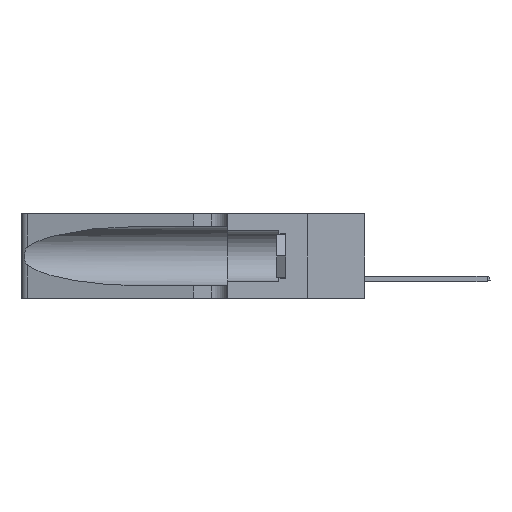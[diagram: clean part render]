
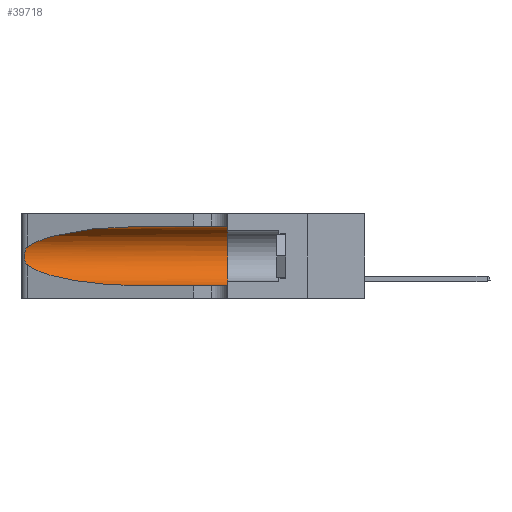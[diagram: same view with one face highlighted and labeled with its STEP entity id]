
A CAD part, left-side view. The second image highlights one B-rep face of the part: STEP entity #39718.
In plain terms, the highlighted cylindrical face has radius 3.308 mm (diameter 6.617 mm), a partial arc.
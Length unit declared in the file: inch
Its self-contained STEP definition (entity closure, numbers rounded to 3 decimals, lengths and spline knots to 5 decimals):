
#500 = VECTOR ( 'NONE', #27007, 39.37008 ) ;
#865 = EDGE_CURVE ( 'NONE', #6688, #7810, #17325, .T. ) ;
#954 = ORIENTED_EDGE ( 'NONE', *, *, #17991, .F. ) ;
#1608 = CARTESIAN_POINT ( 'NONE',  ( 0.1305, 0.72297, 0.05475 ) ) ;
#1954 = ORIENTED_EDGE ( 'NONE', *, *, #3819, .F. ) ;
#2489 = CARTESIAN_POINT ( 'NONE',  ( 0.26018, 1.23835, 0.19895 ) ) ;
#2500 = CARTESIAN_POINT ( 'NONE',  ( 0.1305, 0.72297, 0.31525 ) ) ;
#2977 = CARTESIAN_POINT ( 'NONE',  ( 0.25487, 1.22718, 0.14631 ) ) ;
#3199 = VECTOR ( 'NONE', #20586, 39.37008 ) ;
#3819 = EDGE_CURVE ( 'NONE', #19038, #33625, #8880, .T. ) ;
#3840 = CARTESIAN_POINT ( 'NONE',  ( 0.25487, 1.22718, 0.22369 ) ) ;
#6669 = DIRECTION ( 'NONE',  ( 0., 0., -1. ) ) ;
#6688 = VERTEX_POINT ( 'NONE', #2977 ) ;
#7810 = VERTEX_POINT ( 'NONE', #1608 ) ;
#8698 = CARTESIAN_POINT ( 'NONE',  ( 0.25555, 1.22993, 0.14849 ) ) ;
#8880 = CIRCLE ( 'NONE', #14064, 0.13025 ) ;
#9334 = LINE ( 'NONE', #20278, #500 ) ;
#11957 = CARTESIAN_POINT ( 'NONE',  ( 0.25487, 1.22718, 0.22369 ) ) ;
#11984 = LINE ( 'NONE', #40354, #3199 ) ;
#12287 = CARTESIAN_POINT ( 'NONE',  ( 0.25487, 1.22718, 0.22369 ) ) ;
#13244 = CARTESIAN_POINT ( 'NONE',  ( 0.2373, 1.15595, 0.28018 ) ) ;
#13438 = DIRECTION ( 'NONE',  ( 0., -1., 0. ) ) ;
#14064 = AXIS2_PLACEMENT_3D ( 'NONE', #15494, #18693, #18846 ) ;
#15494 = CARTESIAN_POINT ( 'NONE',  ( 0.1305, 0.35, 0.185 ) ) ;
#15792 = CARTESIAN_POINT ( 'NONE',  ( 0.25555, 1.22994, 0.2215 ) ) ;
#16028 = ORIENTED_EDGE ( 'NONE', *, *, #21395, .T. ) ;
#17325 =( BOUNDED_CURVE ( )  B_SPLINE_CURVE ( 3, ( #21075, #27768, #31559, #21234 ),
 .UNSPECIFIED., .F., .T. ) 
 B_SPLINE_CURVE_WITH_KNOTS ( ( 4, 4 ),
 ( 3.44316, 4.71239 ),
 .UNSPECIFIED. ) 
 CURVE ( )  GEOMETRIC_REPRESENTATION_ITEM ( )  RATIONAL_B_SPLINE_CURVE ( ( 1., 0.87, 0.87, 1. ) ) 
 REPRESENTATION_ITEM ( '' )  );
#17991 = EDGE_CURVE ( 'NONE', #27359, #19038, #11984, .T. ) ;
#18564 = CARTESIAN_POINT ( 'NONE',  ( 0.25854, 1.2359, 0.20912 ) ) ;
#18693 = DIRECTION ( 'NONE',  ( 0., 1., 0. ) ) ;
#18846 = DIRECTION ( 'NONE',  ( 0., 0., 1. ) ) ;
#19038 = VERTEX_POINT ( 'NONE', #35680 ) ;
#19142 = CARTESIAN_POINT ( 'NONE',  ( 0.26075, 1.23896, 0.19203 ) ) ;
#19460 = B_SPLINE_CURVE_WITH_KNOTS ( 'NONE', 3,
 ( #12287, #15792, #22496, #39048, #18564, #2489, #19142, #25429, #25716, #35139, #25276, #28598, #8698, #29026 ),
 .UNSPECIFIED., .F., .F.,
 ( 4, 2, 2, 2, 2, 2, 4 ),
 ( 0., 0.00027, 0.00053, 0.00107, 0.0016, 0.00187, 0.00214 ),
 .UNSPECIFIED. ) ;
#20278 = CARTESIAN_POINT ( 'NONE',  ( 0.1305, 1.61858, 0.05475 ) ) ;
#20586 = DIRECTION ( 'NONE',  ( 0., -1., 0. ) ) ;
#21075 = CARTESIAN_POINT ( 'NONE',  ( 0.25487, 1.22718, 0.14631 ) ) ;
#21234 = CARTESIAN_POINT ( 'NONE',  ( 0.1305, 0.72297, 0.05475 ) ) ;
#21395 = EDGE_CURVE ( 'NONE', #27359, #24284, #21879, .T. ) ;
#21879 =( BOUNDED_CURVE ( )  B_SPLINE_CURVE ( 3, ( #39576, #33212, #13244, #3840 ),
 .UNSPECIFIED., .F., .F. ) 
 B_SPLINE_CURVE_WITH_KNOTS ( ( 4, 4 ),
 ( 1.5708, 2.84003 ),
 .UNSPECIFIED. ) 
 CURVE ( )  GEOMETRIC_REPRESENTATION_ITEM ( )  RATIONAL_B_SPLINE_CURVE ( ( 1., 0.87, 0.87, 1. ) ) 
 REPRESENTATION_ITEM ( '' )  );
#22496 = CARTESIAN_POINT ( 'NONE',  ( 0.25639, 1.23184, 0.21858 ) ) ;
#24284 = VERTEX_POINT ( 'NONE', #11957 ) ;
#25276 = CARTESIAN_POINT ( 'NONE',  ( 0.25789, 1.23486, 0.15765 ) ) ;
#25429 = CARTESIAN_POINT ( 'NONE',  ( 0.26075, 1.23896, 0.178 ) ) ;
#25716 = CARTESIAN_POINT ( 'NONE',  ( 0.26017, 1.23833, 0.17102 ) ) ;
#26080 = ORIENTED_EDGE ( 'NONE', *, *, #865, .T. ) ;
#26978 = ORIENTED_EDGE ( 'NONE', *, *, #42431, .T. ) ;
#27007 = DIRECTION ( 'NONE',  ( 0., -1., 0. ) ) ;
#27359 = VERTEX_POINT ( 'NONE', #2500 ) ;
#27768 = CARTESIAN_POINT ( 'NONE',  ( 0.2373, 1.15595, 0.08982 ) ) ;
#28584 = CYLINDRICAL_SURFACE ( 'NONE', #39801, 0.13025 ) ;
#28598 = CARTESIAN_POINT ( 'NONE',  ( 0.25639, 1.23186, 0.15144 ) ) ;
#29026 = CARTESIAN_POINT ( 'NONE',  ( 0.25487, 1.22718, 0.14631 ) ) ;
#30288 = CARTESIAN_POINT ( 'NONE',  ( 0.1305, 1.61858, 0.185 ) ) ;
#31402 = CARTESIAN_POINT ( 'NONE',  ( 0.1305, 0.35, 0.05475 ) ) ;
#31559 = CARTESIAN_POINT ( 'NONE',  ( 0.18966, 0.96281, 0.05475 ) ) ;
#32856 = EDGE_CURVE ( 'NONE', #7810, #33625, #9334, .T. ) ;
#33212 = CARTESIAN_POINT ( 'NONE',  ( 0.18966, 0.96281, 0.31525 ) ) ;
#33625 = VERTEX_POINT ( 'NONE', #31402 ) ;
#34361 = FACE_OUTER_BOUND ( 'NONE', #39350, .T. ) ;
#35139 = CARTESIAN_POINT ( 'NONE',  ( 0.25856, 1.23593, 0.16098 ) ) ;
#35680 = CARTESIAN_POINT ( 'NONE',  ( 0.1305, 0.35, 0.31525 ) ) ;
#38170 = ORIENTED_EDGE ( 'NONE', *, *, #32856, .T. ) ;
#39048 = CARTESIAN_POINT ( 'NONE',  ( 0.25787, 1.23484, 0.2124 ) ) ;
#39350 = EDGE_LOOP ( 'NONE', ( #16028, #26978, #26080, #38170, #1954, #954 ) ) ;
#39576 = CARTESIAN_POINT ( 'NONE',  ( 0.1305, 0.72297, 0.31525 ) ) ;
#39718 = ADVANCED_FACE ( 'NONE', ( #34361 ), #28584, .F. ) ;
#39801 = AXIS2_PLACEMENT_3D ( 'NONE', #30288, #13438, #6669 ) ;
#40354 = CARTESIAN_POINT ( 'NONE',  ( 0.1305, 1.61858, 0.31525 ) ) ;
#42431 = EDGE_CURVE ( 'NONE', #24284, #6688, #19460, .T. ) ;
